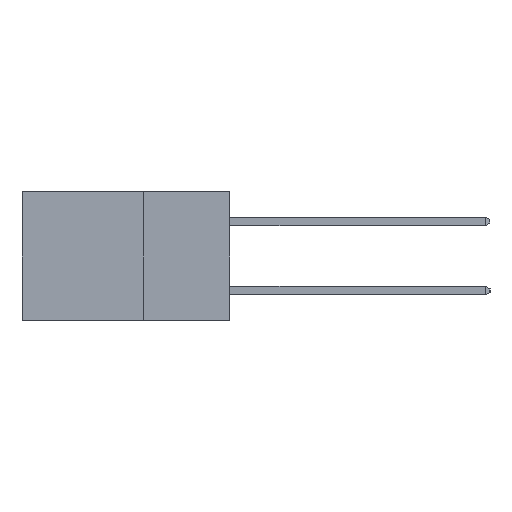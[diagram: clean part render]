
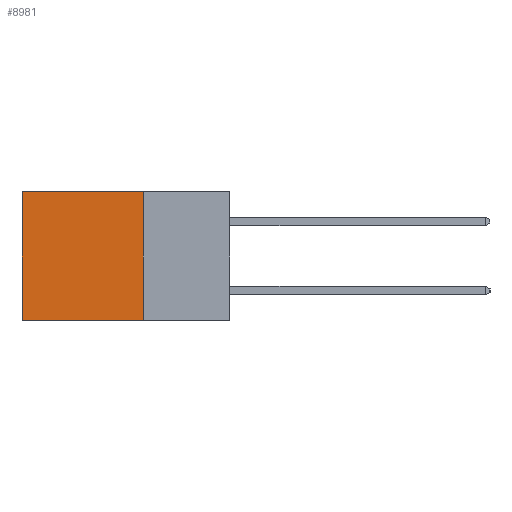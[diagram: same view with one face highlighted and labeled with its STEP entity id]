
A CAD part, left-side view. The second image highlights one B-rep face of the part: STEP entity #8981.
In plain terms, the highlighted planar face has unit normal (-1, 0, 0).
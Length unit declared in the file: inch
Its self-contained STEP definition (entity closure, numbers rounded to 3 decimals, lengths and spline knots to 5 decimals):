
#23 = VECTOR ( 'NONE', #1695, 39.37008 ) ;
#1695 = DIRECTION ( 'NONE',  ( 0., 1., 0. ) ) ;
#1714 = LINE ( 'NONE', #6526, #14144 ) ;
#1802 = CARTESIAN_POINT ( 'NONE',  ( 0.2615, 0.25, -0.37 ) ) ;
#1861 = EDGE_CURVE ( 'NONE', #14163, #12808, #10812, .T. ) ;
#3699 = DIRECTION ( 'NONE',  ( 0., 1., 0. ) ) ;
#3920 = CARTESIAN_POINT ( 'NONE',  ( 0.2615, 0.25, 0. ) ) ;
#4414 = CARTESIAN_POINT ( 'NONE',  ( 0.2615, 0.25, 0. ) ) ;
#4708 = CARTESIAN_POINT ( 'NONE',  ( 0.2615, 0.6, 0. ) ) ;
#4767 = ORIENTED_EDGE ( 'NONE', *, *, #11226, .T. ) ;
#4915 = EDGE_CURVE ( 'NONE', #5161, #13313, #1714, .T. ) ;
#5161 = VERTEX_POINT ( 'NONE', #4414 ) ;
#5444 = EDGE_CURVE ( 'NONE', #13313, #12808, #12735, .T. ) ;
#6053 = FACE_OUTER_BOUND ( 'NONE', #12018, .T. ) ;
#6526 = CARTESIAN_POINT ( 'NONE',  ( 0.2615, 0.25, -0.37 ) ) ;
#6543 = DIRECTION ( 'NONE',  ( 0., 0., -1. ) ) ;
#7153 = DIRECTION ( 'NONE',  ( 0., 0., -1. ) ) ;
#7175 = DIRECTION ( 'NONE',  ( 1., 0., 0. ) ) ;
#7180 = PLANE ( 'NONE',  #13309 ) ;
#7445 = CARTESIAN_POINT ( 'NONE',  ( 0.2615, 0.25, -0.37 ) ) ;
#8427 = ORIENTED_EDGE ( 'NONE', *, *, #5444, .F. ) ;
#8483 = VECTOR ( 'NONE', #3699, 39.37008 ) ;
#8882 = LINE ( 'NONE', #3920, #8483 ) ;
#8981 = ADVANCED_FACE ( 'NONE', ( #6053 ), #7180, .F. ) ;
#10498 = ORIENTED_EDGE ( 'NONE', *, *, #1861, .T. ) ;
#10812 = LINE ( 'NONE', #14229, #13873 ) ;
#11226 = EDGE_CURVE ( 'NONE', #5161, #14163, #8882, .T. ) ;
#11365 = CARTESIAN_POINT ( 'NONE',  ( 0.2615, 0.25, -0.37 ) ) ;
#11975 = ORIENTED_EDGE ( 'NONE', *, *, #4915, .F. ) ;
#12018 = EDGE_LOOP ( 'NONE', ( #10498, #8427, #11975, #4767 ) ) ;
#12591 = DIRECTION ( 'NONE',  ( 0., 0., -1. ) ) ;
#12735 = LINE ( 'NONE', #1802, #23 ) ;
#12808 = VERTEX_POINT ( 'NONE', #15033 ) ;
#13309 = AXIS2_PLACEMENT_3D ( 'NONE', #7445, #7175, #7153 ) ;
#13313 = VERTEX_POINT ( 'NONE', #11365 ) ;
#13873 = VECTOR ( 'NONE', #12591, 39.37008 ) ;
#14144 = VECTOR ( 'NONE', #6543, 39.37008 ) ;
#14163 = VERTEX_POINT ( 'NONE', #4708 ) ;
#14229 = CARTESIAN_POINT ( 'NONE',  ( 0.2615, 0.6, -0.37 ) ) ;
#15033 = CARTESIAN_POINT ( 'NONE',  ( 0.2615, 0.6, -0.37 ) ) ;
